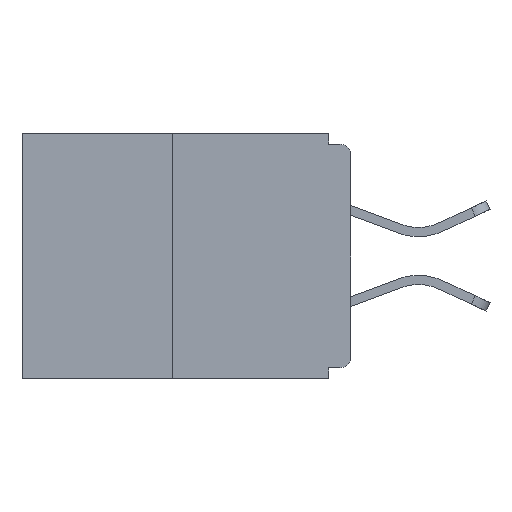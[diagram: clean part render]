
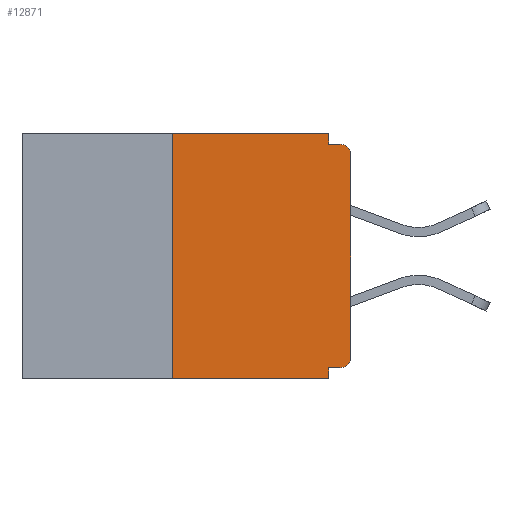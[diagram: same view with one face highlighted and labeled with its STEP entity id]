
A CAD part, left-side view. The second image highlights one B-rep face of the part: STEP entity #12871.
In plain terms, the highlighted planar face has unit normal (-1, 0, 0).
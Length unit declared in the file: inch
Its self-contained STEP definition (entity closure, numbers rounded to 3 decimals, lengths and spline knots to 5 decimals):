
#69 = PLANE ( 'NONE',  #20504 ) ;
#237 = VECTOR ( 'NONE', #25741, 39.37008 ) ;
#397 = CARTESIAN_POINT ( 'NONE',  ( 0., 0.46, 0. ) ) ;
#978 = ORIENTED_EDGE ( 'NONE', *, *, #25684, .F. ) ;
#1219 = VERTEX_POINT ( 'NONE', #5582 ) ;
#1379 = EDGE_CURVE ( 'NONE', #12713, #2296, #11767, .T. ) ;
#1398 = CARTESIAN_POINT ( 'NONE',  ( 0., 0.031, -0.343 ) ) ;
#1718 = DIRECTION ( 'NONE',  ( 0., 1., 0. ) ) ;
#1811 = VECTOR ( 'NONE', #27667, 39.37008 ) ;
#1898 = AXIS2_PLACEMENT_3D ( 'NONE', #27375, #3618, #10355 ) ;
#2250 = CARTESIAN_POINT ( 'NONE',  ( 0., 0., -0.03 ) ) ;
#2296 = VERTEX_POINT ( 'NONE', #6461 ) ;
#2374 = ORIENTED_EDGE ( 'NONE', *, *, #1379, .F. ) ;
#2487 = AXIS2_PLACEMENT_3D ( 'NONE', #9799, #19690, #2767 ) ;
#2767 = DIRECTION ( 'NONE',  ( 0., 0., -1. ) ) ;
#3301 = CARTESIAN_POINT ( 'NONE',  ( 0., 0.25, 0. ) ) ;
#3618 = DIRECTION ( 'NONE',  ( -1., 0., 0. ) ) ;
#3695 = VECTOR ( 'NONE', #10666, 39.37008 ) ;
#4034 = VECTOR ( 'NONE', #1718, 39.37008 ) ;
#4744 = EDGE_CURVE ( 'NONE', #18470, #10970, #21656, .T. ) ;
#4801 = CARTESIAN_POINT ( 'NONE',  ( 0., 0., -0.015 ) ) ;
#5412 = ORIENTED_EDGE ( 'NONE', *, *, #15554, .T. ) ;
#5574 = DIRECTION ( 'NONE',  ( 0., 0., -1. ) ) ;
#5582 = CARTESIAN_POINT ( 'NONE',  ( 0., 0.25, 0. ) ) ;
#5655 = VERTEX_POINT ( 'NONE', #12602 ) ;
#5846 = VERTEX_POINT ( 'NONE', #29458 ) ;
#6264 = LINE ( 'NONE', #27561, #4034 ) ;
#6461 = CARTESIAN_POINT ( 'NONE',  ( 0., 0.031, -0.015 ) ) ;
#6676 = CARTESIAN_POINT ( 'NONE',  ( 0., 0.015, -0.015 ) ) ;
#7221 = DIRECTION ( 'NONE',  ( 0., 0., -1. ) ) ;
#8662 = CARTESIAN_POINT ( 'NONE',  ( 0., 0.46, 0. ) ) ;
#9594 = LINE ( 'NONE', #8662, #1811 ) ;
#9799 = CARTESIAN_POINT ( 'NONE',  ( 0., 0.015, -0.03 ) ) ;
#9882 = VECTOR ( 'NONE', #5574, 39.37008 ) ;
#10063 = VECTOR ( 'NONE', #26540, 39.37008 ) ;
#10355 = DIRECTION ( 'NONE',  ( 0., 0., -1. ) ) ;
#10400 = ORIENTED_EDGE ( 'NONE', *, *, #16113, .F. ) ;
#10595 = LINE ( 'NONE', #27846, #237 ) ;
#10666 = DIRECTION ( 'NONE',  ( 0., -1., 0. ) ) ;
#10970 = VERTEX_POINT ( 'NONE', #28716 ) ;
#11050 = EDGE_CURVE ( 'NONE', #19941, #1219, #16375, .T. ) ;
#11767 = LINE ( 'NONE', #24051, #9882 ) ;
#12602 = CARTESIAN_POINT ( 'NONE',  ( 0., 0.031, -0.328 ) ) ;
#12649 = EDGE_CURVE ( 'NONE', #18470, #5655, #6264, .T. ) ;
#12713 = VERTEX_POINT ( 'NONE', #17043 ) ;
#12871 = ADVANCED_FACE ( 'NONE', ( #30329 ), #69, .F. ) ;
#12951 = CARTESIAN_POINT ( 'NONE',  ( 0., 0.015, -0.328 ) ) ;
#13472 = ORIENTED_EDGE ( 'NONE', *, *, #11050, .F. ) ;
#13575 = LINE ( 'NONE', #4801, #24358 ) ;
#14304 = EDGE_CURVE ( 'NONE', #19941, #5846, #18152, .T. ) ;
#14452 = VERTEX_POINT ( 'NONE', #2250 ) ;
#15283 = CARTESIAN_POINT ( 'NONE',  ( 0., 0.25, -0.343 ) ) ;
#15554 = EDGE_CURVE ( 'NONE', #14452, #23928, #21810, .T. ) ;
#16113 = EDGE_CURVE ( 'NONE', #2296, #23928, #13575, .T. ) ;
#16375 = LINE ( 'NONE', #3301, #10063 ) ;
#17043 = CARTESIAN_POINT ( 'NONE',  ( 0., 0.031, 0. ) ) ;
#17563 = EDGE_LOOP ( 'NONE', ( #19096, #13472, #25240, #978, #28675, #20013, #27521, #5412, #10400, #2374 ) ) ;
#17925 = CARTESIAN_POINT ( 'NONE',  ( 0., 0.46, -0.343 ) ) ;
#18152 = LINE ( 'NONE', #17925, #3695 ) ;
#18470 = VERTEX_POINT ( 'NONE', #12951 ) ;
#19056 = DIRECTION ( 'NONE',  ( 1., 0., 0. ) ) ;
#19071 = EDGE_CURVE ( 'NONE', #10970, #14452, #10595, .T. ) ;
#19096 = ORIENTED_EDGE ( 'NONE', *, *, #29163, .F. ) ;
#19690 = DIRECTION ( 'NONE',  ( -1., 0., 0. ) ) ;
#19768 = DIRECTION ( 'NONE',  ( 0., 0., -1. ) ) ;
#19941 = VERTEX_POINT ( 'NONE', #15283 ) ;
#20013 = ORIENTED_EDGE ( 'NONE', *, *, #4744, .T. ) ;
#20504 = AXIS2_PLACEMENT_3D ( 'NONE', #397, #19056, #7221 ) ;
#21656 = CIRCLE ( 'NONE', #1898, 0.015 ) ;
#21810 = CIRCLE ( 'NONE', #2487, 0.015 ) ;
#23165 = LINE ( 'NONE', #1398, #30207 ) ;
#23790 = DIRECTION ( 'NONE',  ( 0., -1., 0. ) ) ;
#23928 = VERTEX_POINT ( 'NONE', #6676 ) ;
#24051 = CARTESIAN_POINT ( 'NONE',  ( 0., 0.031, 0. ) ) ;
#24358 = VECTOR ( 'NONE', #23790, 39.37008 ) ;
#25240 = ORIENTED_EDGE ( 'NONE', *, *, #14304, .T. ) ;
#25684 = EDGE_CURVE ( 'NONE', #5655, #5846, #23165, .T. ) ;
#25741 = DIRECTION ( 'NONE',  ( 0., 0., 1. ) ) ;
#26540 = DIRECTION ( 'NONE',  ( 0., 0., 1. ) ) ;
#27375 = CARTESIAN_POINT ( 'NONE',  ( 0., 0.015, -0.313 ) ) ;
#27521 = ORIENTED_EDGE ( 'NONE', *, *, #19071, .T. ) ;
#27561 = CARTESIAN_POINT ( 'NONE',  ( 0., 0., -0.328 ) ) ;
#27667 = DIRECTION ( 'NONE',  ( 0., -1., 0. ) ) ;
#27846 = CARTESIAN_POINT ( 'NONE',  ( 0., 0., 0. ) ) ;
#28675 = ORIENTED_EDGE ( 'NONE', *, *, #12649, .F. ) ;
#28716 = CARTESIAN_POINT ( 'NONE',  ( 0., 0., -0.313 ) ) ;
#29163 = EDGE_CURVE ( 'NONE', #1219, #12713, #9594, .T. ) ;
#29458 = CARTESIAN_POINT ( 'NONE',  ( 0., 0.031, -0.343 ) ) ;
#30207 = VECTOR ( 'NONE', #19768, 39.37008 ) ;
#30329 = FACE_OUTER_BOUND ( 'NONE', #17563, .T. ) ;
